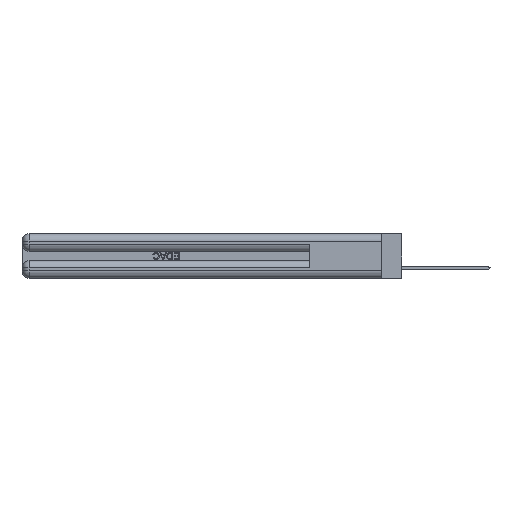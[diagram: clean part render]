
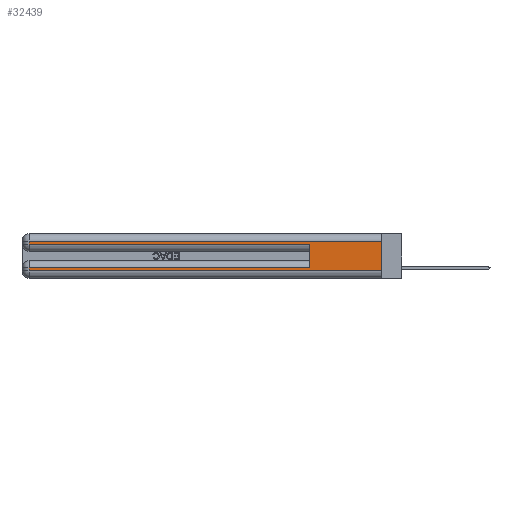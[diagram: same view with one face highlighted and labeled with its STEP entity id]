
A CAD part, left-side view. The second image highlights one B-rep face of the part: STEP entity #32439.
In plain terms, the highlighted planar face has unit normal (-1, 0, 0).
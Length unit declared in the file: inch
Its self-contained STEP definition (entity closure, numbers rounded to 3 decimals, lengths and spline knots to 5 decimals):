
#84 = ORIENTED_EDGE ( 'NONE', *, *, #30005, .T. ) ;
#220 = VECTOR ( 'NONE', #48456, 39.37008 ) ;
#754 = DIRECTION ( 'NONE',  ( 0., 1., 0. ) ) ;
#2059 = VECTOR ( 'NONE', #754, 39.37008 ) ;
#2354 = DIRECTION ( 'NONE',  ( 0., 0., -1. ) ) ;
#2398 = CARTESIAN_POINT ( 'NONE',  ( 0., 2.94, 0.285 ) ) ;
#5109 = CARTESIAN_POINT ( 'NONE',  ( 0., 0., 0.285 ) ) ;
#6965 = EDGE_CURVE ( 'NONE', #40803, #33301, #34374, .T. ) ;
#8647 = LINE ( 'NONE', #10395, #39999 ) ;
#10198 = CARTESIAN_POINT ( 'NONE',  ( 0., 0.6, 0.085 ) ) ;
#10395 = CARTESIAN_POINT ( 'NONE',  ( 0., 0., 0.37 ) ) ;
#11424 = DIRECTION ( 'NONE',  ( 0., -1., 0. ) ) ;
#11545 = VERTEX_POINT ( 'NONE', #17674 ) ;
#11993 = PLANE ( 'NONE',  #42149 ) ;
#12211 = DIRECTION ( 'NONE',  ( 0., 0., -1. ) ) ;
#12324 = LINE ( 'NONE', #33881, #2059 ) ;
#13981 = VERTEX_POINT ( 'NONE', #10198 ) ;
#14378 = DIRECTION ( 'NONE',  ( 0., 0., -1. ) ) ;
#16098 = VERTEX_POINT ( 'NONE', #48677 ) ;
#17159 = DIRECTION ( 'NONE',  ( 0., 0., 1. ) ) ;
#17674 = CARTESIAN_POINT ( 'NONE',  ( 0., 2.94, 0.06 ) ) ;
#18328 = LINE ( 'NONE', #34463, #48306 ) ;
#20743 = ORIENTED_EDGE ( 'NONE', *, *, #33377, .T. ) ;
#21071 = ORIENTED_EDGE ( 'NONE', *, *, #51748, .F. ) ;
#21512 = VECTOR ( 'NONE', #17159, 39.37008 ) ;
#21772 = CARTESIAN_POINT ( 'NONE',  ( 0., 2.94, 0.085 ) ) ;
#22668 = VERTEX_POINT ( 'NONE', #28020 ) ;
#25835 = EDGE_CURVE ( 'NONE', #11545, #16098, #18328, .T. ) ;
#25865 = ORIENTED_EDGE ( 'NONE', *, *, #27387, .T. ) ;
#27387 = EDGE_CURVE ( 'NONE', #22668, #40803, #51018, .T. ) ;
#28020 = CARTESIAN_POINT ( 'NONE',  ( 0., 2.94, 0.31 ) ) ;
#28363 = CARTESIAN_POINT ( 'NONE',  ( 0., 2.94, 0.37 ) ) ;
#28715 = ORIENTED_EDGE ( 'NONE', *, *, #25835, .T. ) ;
#30005 = EDGE_CURVE ( 'NONE', #51622, #11545, #48851, .T. ) ;
#30397 = EDGE_CURVE ( 'NONE', #49055, #22668, #31672, .T. ) ;
#31672 = LINE ( 'NONE', #43879, #220 ) ;
#32439 = ADVANCED_FACE ( 'NONE', ( #45561 ), #11993, .F. ) ;
#33301 = VERTEX_POINT ( 'NONE', #47976 ) ;
#33377 = EDGE_CURVE ( 'NONE', #13981, #51622, #12324, .T. ) ;
#33629 = DIRECTION ( 'NONE',  ( 0., 0., -1. ) ) ;
#33881 = CARTESIAN_POINT ( 'NONE',  ( 0., 0., 0.085 ) ) ;
#34374 = LINE ( 'NONE', #5109, #36960 ) ;
#34463 = CARTESIAN_POINT ( 'NONE',  ( 0., 0., 0.06 ) ) ;
#34766 = DIRECTION ( 'NONE',  ( 1., 0., 0. ) ) ;
#35145 = ORIENTED_EDGE ( 'NONE', *, *, #6965, .T. ) ;
#35990 = ORIENTED_EDGE ( 'NONE', *, *, #30397, .T. ) ;
#36960 = VECTOR ( 'NONE', #11424, 39.37008 ) ;
#37992 = VECTOR ( 'NONE', #14378, 39.37008 ) ;
#39999 = VECTOR ( 'NONE', #2354, 39.37008 ) ;
#40803 = VERTEX_POINT ( 'NONE', #2398 ) ;
#41728 = CARTESIAN_POINT ( 'NONE',  ( 0., 0., 0.31 ) ) ;
#42149 = AXIS2_PLACEMENT_3D ( 'NONE', #46099, #34766, #12211 ) ;
#42801 = DIRECTION ( 'NONE',  ( 0., -1., 0. ) ) ;
#43658 = EDGE_CURVE ( 'NONE', #13981, #33301, #52811, .T. ) ;
#43879 = CARTESIAN_POINT ( 'NONE',  ( 0., 0., 0.31 ) ) ;
#45372 = CARTESIAN_POINT ( 'NONE',  ( 0., 2.94, 0.37 ) ) ;
#45561 = FACE_OUTER_BOUND ( 'NONE', #52375, .T. ) ;
#46099 = CARTESIAN_POINT ( 'NONE',  ( 0., 0., 0.37 ) ) ;
#47976 = CARTESIAN_POINT ( 'NONE',  ( 0., 0.6, 0.285 ) ) ;
#48306 = VECTOR ( 'NONE', #42801, 39.37008 ) ;
#48456 = DIRECTION ( 'NONE',  ( 0., 1., 0. ) ) ;
#48677 = CARTESIAN_POINT ( 'NONE',  ( 0., 0., 0.06 ) ) ;
#48851 = LINE ( 'NONE', #45372, #37992 ) ;
#49055 = VERTEX_POINT ( 'NONE', #41728 ) ;
#49404 = CARTESIAN_POINT ( 'NONE',  ( 0., 0.6, 0.145 ) ) ;
#51018 = LINE ( 'NONE', #28363, #51692 ) ;
#51422 = ORIENTED_EDGE ( 'NONE', *, *, #43658, .F. ) ;
#51622 = VERTEX_POINT ( 'NONE', #21772 ) ;
#51692 = VECTOR ( 'NONE', #33629, 39.37008 ) ;
#51748 = EDGE_CURVE ( 'NONE', #49055, #16098, #8647, .T. ) ;
#52375 = EDGE_LOOP ( 'NONE', ( #21071, #35990, #25865, #35145, #51422, #20743, #84, #28715 ) ) ;
#52811 = LINE ( 'NONE', #49404, #21512 ) ;
